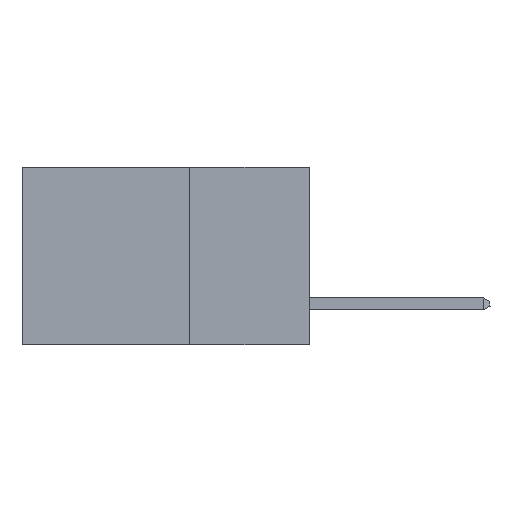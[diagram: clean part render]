
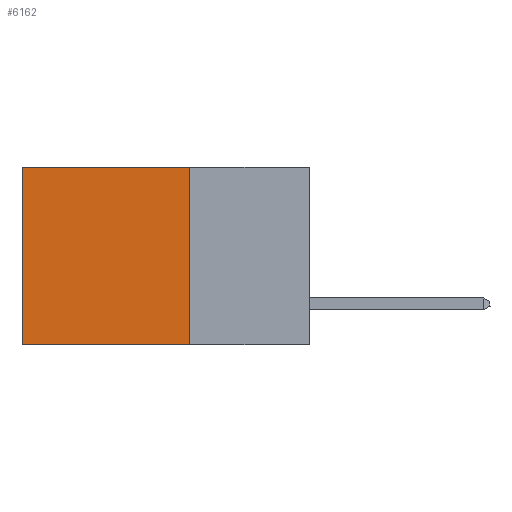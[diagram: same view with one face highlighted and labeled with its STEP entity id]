
A CAD part, left-side view. The second image highlights one B-rep face of the part: STEP entity #6162.
In plain terms, the highlighted planar face has unit normal (-1, 0, 0).
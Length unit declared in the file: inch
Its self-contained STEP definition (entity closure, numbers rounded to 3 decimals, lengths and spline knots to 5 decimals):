
#839 = PLANE ( 'NONE',  #19457 ) ;
#1212 = LINE ( 'NONE', #20459, #33159 ) ;
#2113 = CARTESIAN_POINT ( 'NONE',  ( 0.2875, 0.6, -0.37 ) ) ;
#2655 = LINE ( 'NONE', #35193, #6442 ) ;
#4174 = DIRECTION ( 'NONE',  ( 0., 0., -1. ) ) ;
#4208 = FACE_OUTER_BOUND ( 'NONE', #9404, .T. ) ;
#5251 = EDGE_CURVE ( 'NONE', #24605, #24727, #30072, .T. ) ;
#5279 = ORIENTED_EDGE ( 'NONE', *, *, #24819, .F. ) ;
#6162 = ADVANCED_FACE ( 'NONE', ( #4208 ), #839, .F. ) ;
#6249 = VECTOR ( 'NONE', #25546, 39.37008 ) ;
#6442 = VECTOR ( 'NONE', #21550, 39.37008 ) ;
#9404 = EDGE_LOOP ( 'NONE', ( #16765, #31063, #5279, #30168 ) ) ;
#10064 = CARTESIAN_POINT ( 'NONE',  ( 0.2875, 0.25, 0. ) ) ;
#11628 = VECTOR ( 'NONE', #28777, 39.37008 ) ;
#13852 = VERTEX_POINT ( 'NONE', #25563 ) ;
#16765 = ORIENTED_EDGE ( 'NONE', *, *, #19449, .T. ) ;
#17290 = LINE ( 'NONE', #10064, #6249 ) ;
#17597 = CARTESIAN_POINT ( 'NONE',  ( 0.2875, 0.25, -0.37 ) ) ;
#17665 = DIRECTION ( 'NONE',  ( 1., 0., 0. ) ) ;
#19449 = EDGE_CURVE ( 'NONE', #33245, #24727, #1212, .T. ) ;
#19457 = AXIS2_PLACEMENT_3D ( 'NONE', #28202, #17665, #30909 ) ;
#19722 = CARTESIAN_POINT ( 'NONE',  ( 0.2875, 0.6, 0. ) ) ;
#20459 = CARTESIAN_POINT ( 'NONE',  ( 0.2875, 0.6, 0. ) ) ;
#21550 = DIRECTION ( 'NONE',  ( 0., 1., 0. ) ) ;
#24605 = VERTEX_POINT ( 'NONE', #17597 ) ;
#24727 = VERTEX_POINT ( 'NONE', #2113 ) ;
#24819 = EDGE_CURVE ( 'NONE', #13852, #24605, #17290, .T. ) ;
#25546 = DIRECTION ( 'NONE',  ( 0., 0., -1. ) ) ;
#25563 = CARTESIAN_POINT ( 'NONE',  ( 0.2875, 0.25, 0. ) ) ;
#27982 = EDGE_CURVE ( 'NONE', #13852, #33245, #2655, .T. ) ;
#28202 = CARTESIAN_POINT ( 'NONE',  ( 0.2875, 0.25, 0. ) ) ;
#28777 = DIRECTION ( 'NONE',  ( 0., 1., 0. ) ) ;
#30072 = LINE ( 'NONE', #31176, #11628 ) ;
#30168 = ORIENTED_EDGE ( 'NONE', *, *, #27982, .T. ) ;
#30909 = DIRECTION ( 'NONE',  ( 0., 0., -1. ) ) ;
#31063 = ORIENTED_EDGE ( 'NONE', *, *, #5251, .F. ) ;
#31176 = CARTESIAN_POINT ( 'NONE',  ( 0.2875, 0.25, -0.37 ) ) ;
#33159 = VECTOR ( 'NONE', #4174, 39.37008 ) ;
#33245 = VERTEX_POINT ( 'NONE', #19722 ) ;
#35193 = CARTESIAN_POINT ( 'NONE',  ( 0.2875, 0.25, 0. ) ) ;
